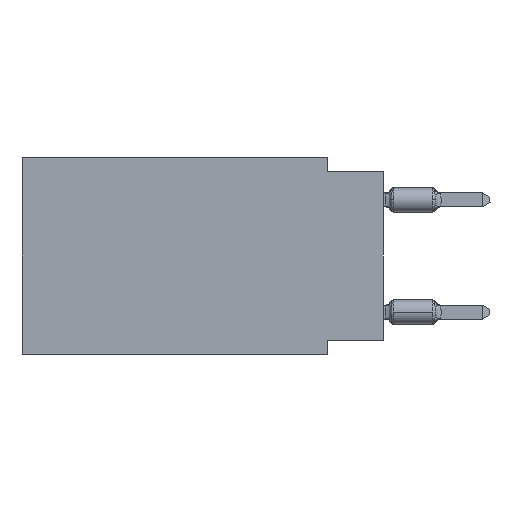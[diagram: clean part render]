
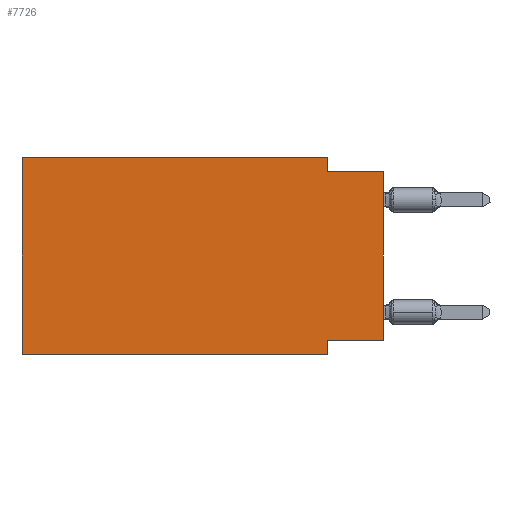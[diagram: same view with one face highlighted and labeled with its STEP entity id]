
A CAD part, left-side view. The second image highlights one B-rep face of the part: STEP entity #7726.
In plain terms, the highlighted planar face has unit normal (-1, 0, 0).
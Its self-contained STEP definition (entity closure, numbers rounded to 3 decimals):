
#123 = ORIENTED_EDGE ( 'NONE', *, *, #8152, .F. ) ;
#480 = EDGE_CURVE ( 'NONE', #15128, #9777, #2064, .T. ) ;
#692 = VERTEX_POINT ( 'NONE', #1645 ) ;
#972 = CARTESIAN_POINT ( 'NONE',  ( 0., 0., -0.635 ) ) ;
#1273 = EDGE_CURVE ( 'NONE', #692, #23432, #17710, .T. ) ;
#1645 = CARTESIAN_POINT ( 'NONE',  ( 0., 0., -8.255 ) ) ;
#2064 = LINE ( 'NONE', #9690, #21098 ) ;
#2226 = DIRECTION ( 'NONE',  ( 0., 1., 0. ) ) ;
#3277 = DIRECTION ( 'NONE',  ( 0., 0., -1. ) ) ;
#3306 = LINE ( 'NONE', #18543, #20957 ) ;
#3803 = CARTESIAN_POINT ( 'NONE',  ( 0., 2.54, -8.255 ) ) ;
#3808 = CARTESIAN_POINT ( 'NONE',  ( 0., 2.54, 0. ) ) ;
#4071 = DIRECTION ( 'NONE',  ( 0., -1., 0. ) ) ;
#5127 = ORIENTED_EDGE ( 'NONE', *, *, #480, .T. ) ;
#5308 = DIRECTION ( 'NONE',  ( 0., 0., 1. ) ) ;
#6543 = ORIENTED_EDGE ( 'NONE', *, *, #1273, .F. ) ;
#6990 = VECTOR ( 'NONE', #13717, 1000. ) ;
#7634 = EDGE_LOOP ( 'NONE', ( #11758, #123, #20041, #22257, #13982, #5127, #11078, #6543 ) ) ;
#7726 = ADVANCED_FACE ( 'NONE', ( #22743 ), #14882, .F. ) ;
#8152 = EDGE_CURVE ( 'NONE', #18735, #11685, #14851, .T. ) ;
#9690 = CARTESIAN_POINT ( 'NONE',  ( 0., 16.383, -8.89 ) ) ;
#9716 = VECTOR ( 'NONE', #12977, 1000. ) ;
#9777 = VERTEX_POINT ( 'NONE', #13196 ) ;
#10208 = VECTOR ( 'NONE', #5308, 1000. ) ;
#10369 = CARTESIAN_POINT ( 'NONE',  ( 0., 16.383, 0. ) ) ;
#10768 = AXIS2_PLACEMENT_3D ( 'NONE', #20506, #22379, #3277 ) ;
#10984 = DIRECTION ( 'NONE',  ( 0., 0., 1. ) ) ;
#11078 = ORIENTED_EDGE ( 'NONE', *, *, #18163, .F. ) ;
#11683 = CARTESIAN_POINT ( 'NONE',  ( 0., 16.383, 0. ) ) ;
#11685 = VERTEX_POINT ( 'NONE', #972 ) ;
#11758 = ORIENTED_EDGE ( 'NONE', *, *, #17048, .T. ) ;
#12842 = LINE ( 'NONE', #20462, #21873 ) ;
#12977 = DIRECTION ( 'NONE',  ( 0., -1., 0. ) ) ;
#13196 = CARTESIAN_POINT ( 'NONE',  ( 0., 2.54, -8.89 ) ) ;
#13468 = EDGE_CURVE ( 'NONE', #24556, #18735, #3306, .T. ) ;
#13536 = EDGE_CURVE ( 'NONE', #15128, #18840, #22407, .T. ) ;
#13717 = DIRECTION ( 'NONE',  ( 0., -1., 0. ) ) ;
#13982 = ORIENTED_EDGE ( 'NONE', *, *, #13536, .F. ) ;
#14761 = VECTOR ( 'NONE', #19144, 1000. ) ;
#14851 = LINE ( 'NONE', #16605, #9716 ) ;
#14882 = PLANE ( 'NONE',  #10768 ) ;
#15128 = VERTEX_POINT ( 'NONE', #17115 ) ;
#16605 = CARTESIAN_POINT ( 'NONE',  ( 0., 0., -0.635 ) ) ;
#17048 = EDGE_CURVE ( 'NONE', #692, #11685, #12842, .T. ) ;
#17115 = CARTESIAN_POINT ( 'NONE',  ( 0., 16.383, -8.89 ) ) ;
#17710 = LINE ( 'NONE', #17836, #24319 ) ;
#17836 = CARTESIAN_POINT ( 'NONE',  ( 0., 0., -8.255 ) ) ;
#18163 = EDGE_CURVE ( 'NONE', #23432, #9777, #23002, .T. ) ;
#18543 = CARTESIAN_POINT ( 'NONE',  ( 0., 2.54, 0. ) ) ;
#18689 = CARTESIAN_POINT ( 'NONE',  ( 0., 2.54, -0.635 ) ) ;
#18735 = VERTEX_POINT ( 'NONE', #18689 ) ;
#18840 = VERTEX_POINT ( 'NONE', #11683 ) ;
#19144 = DIRECTION ( 'NONE',  ( 0., 0., -1. ) ) ;
#19349 = LINE ( 'NONE', #10369, #6990 ) ;
#19508 = CARTESIAN_POINT ( 'NONE',  ( 0., 2.54, -8.89 ) ) ;
#20041 = ORIENTED_EDGE ( 'NONE', *, *, #13468, .F. ) ;
#20462 = CARTESIAN_POINT ( 'NONE',  ( 0., 0., 0. ) ) ;
#20506 = CARTESIAN_POINT ( 'NONE',  ( 0., 16.383, 0. ) ) ;
#20894 = CARTESIAN_POINT ( 'NONE',  ( 0., 16.383, 0. ) ) ;
#20957 = VECTOR ( 'NONE', #22531, 1000. ) ;
#21098 = VECTOR ( 'NONE', #4071, 1000. ) ;
#21799 = EDGE_CURVE ( 'NONE', #18840, #24556, #19349, .T. ) ;
#21873 = VECTOR ( 'NONE', #10984, 1000. ) ;
#22257 = ORIENTED_EDGE ( 'NONE', *, *, #21799, .F. ) ;
#22379 = DIRECTION ( 'NONE',  ( 1., 0., 0. ) ) ;
#22407 = LINE ( 'NONE', #20894, #10208 ) ;
#22531 = DIRECTION ( 'NONE',  ( 0., 0., -1. ) ) ;
#22743 = FACE_OUTER_BOUND ( 'NONE', #7634, .T. ) ;
#23002 = LINE ( 'NONE', #19508, #14761 ) ;
#23432 = VERTEX_POINT ( 'NONE', #3803 ) ;
#24319 = VECTOR ( 'NONE', #2226, 1000. ) ;
#24556 = VERTEX_POINT ( 'NONE', #3808 ) ;
